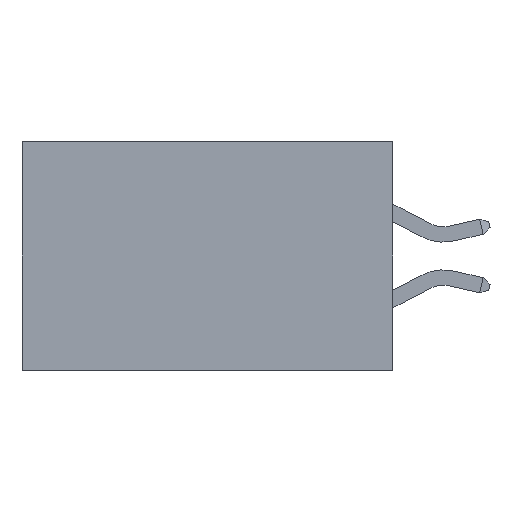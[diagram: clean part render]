
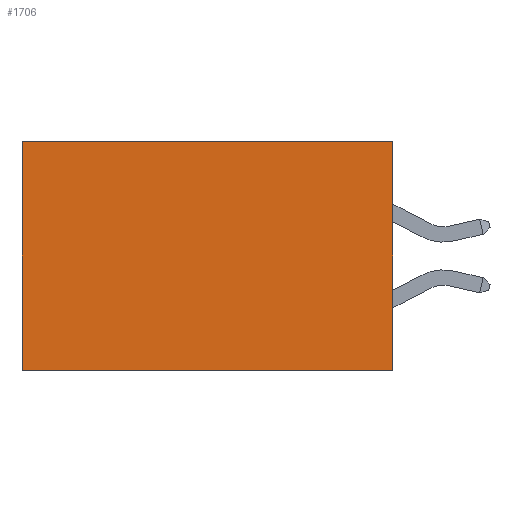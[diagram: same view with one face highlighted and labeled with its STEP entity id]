
A CAD part, left-side view. The second image highlights one B-rep face of the part: STEP entity #1706.
In plain terms, the highlighted planar face has unit normal (-1, 0, 0).
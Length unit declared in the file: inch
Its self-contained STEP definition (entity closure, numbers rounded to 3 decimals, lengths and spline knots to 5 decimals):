
#2 = DIRECTION ( 'NONE',  ( 0., 0., -1. ) ) ;
#675 = DIRECTION ( 'NONE',  ( 0., 0., -1. ) ) ;
#712 = CARTESIAN_POINT ( 'NONE',  ( 0.2875, 0.6, 0. ) ) ;
#774 = EDGE_CURVE ( 'NONE', #2079, #1591, #3200, .T. ) ;
#822 = ORIENTED_EDGE ( 'NONE', *, *, #8198, .F. ) ;
#846 = ORIENTED_EDGE ( 'NONE', *, *, #774, .T. ) ;
#1236 = EDGE_CURVE ( 'NONE', #7337, #1591, #2069, .T. ) ;
#1397 = LINE ( 'NONE', #6711, #5635 ) ;
#1412 = LINE ( 'NONE', #6816, #7905 ) ;
#1591 = VERTEX_POINT ( 'NONE', #10104 ) ;
#1613 = VERTEX_POINT ( 'NONE', #3471 ) ;
#1706 = ADVANCED_FACE ( 'NONE', ( #8808 ), #4520, .F. ) ;
#2033 = ORIENTED_EDGE ( 'NONE', *, *, #1236, .F. ) ;
#2069 = LINE ( 'NONE', #2232, #6125 ) ;
#2079 = VERTEX_POINT ( 'NONE', #2326 ) ;
#2232 = CARTESIAN_POINT ( 'NONE',  ( 0.2875, 0., -0.37 ) ) ;
#2326 = CARTESIAN_POINT ( 'NONE',  ( 0.2875, 0.6, 0. ) ) ;
#3200 = LINE ( 'NONE', #712, #7160 ) ;
#3471 = CARTESIAN_POINT ( 'NONE',  ( 0.2875, 0., 0. ) ) ;
#3529 = EDGE_LOOP ( 'NONE', ( #846, #2033, #822, #6643 ) ) ;
#3925 = DIRECTION ( 'NONE',  ( 0., 1., 0. ) ) ;
#4051 = EDGE_CURVE ( 'NONE', #1613, #2079, #1412, .T. ) ;
#4520 = PLANE ( 'NONE',  #4992 ) ;
#4992 = AXIS2_PLACEMENT_3D ( 'NONE', #6247, #5405, #5417 ) ;
#5405 = DIRECTION ( 'NONE',  ( 1., 0., 0. ) ) ;
#5417 = DIRECTION ( 'NONE',  ( 0., 0., -1. ) ) ;
#5635 = VECTOR ( 'NONE', #2, 39.37008 ) ;
#6125 = VECTOR ( 'NONE', #3925, 39.37008 ) ;
#6247 = CARTESIAN_POINT ( 'NONE',  ( 0.2875, 0., 0. ) ) ;
#6643 = ORIENTED_EDGE ( 'NONE', *, *, #4051, .T. ) ;
#6711 = CARTESIAN_POINT ( 'NONE',  ( 0.2875, 0., 0. ) ) ;
#6816 = CARTESIAN_POINT ( 'NONE',  ( 0.2875, 0., 0. ) ) ;
#7160 = VECTOR ( 'NONE', #675, 39.37008 ) ;
#7251 = CARTESIAN_POINT ( 'NONE',  ( 0.2875, 0., -0.37 ) ) ;
#7337 = VERTEX_POINT ( 'NONE', #7251 ) ;
#7905 = VECTOR ( 'NONE', #7983, 39.37008 ) ;
#7983 = DIRECTION ( 'NONE',  ( 0., 1., 0. ) ) ;
#8198 = EDGE_CURVE ( 'NONE', #1613, #7337, #1397, .T. ) ;
#8808 = FACE_OUTER_BOUND ( 'NONE', #3529, .T. ) ;
#10104 = CARTESIAN_POINT ( 'NONE',  ( 0.2875, 0.6, -0.37 ) ) ;
